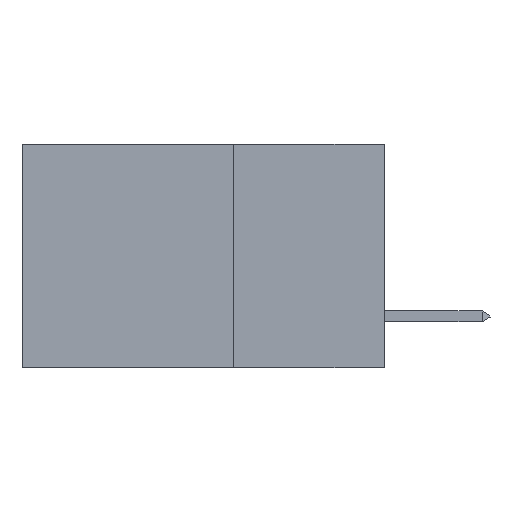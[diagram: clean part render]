
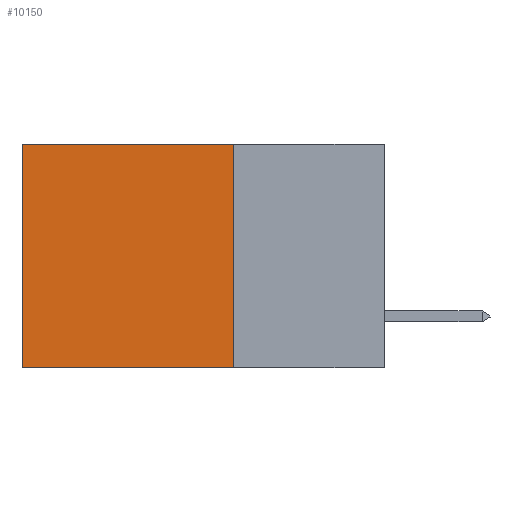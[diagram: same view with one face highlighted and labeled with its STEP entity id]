
A CAD part, left-side view. The second image highlights one B-rep face of the part: STEP entity #10150.
In plain terms, the highlighted planar face has unit normal (-1, 0, 0).
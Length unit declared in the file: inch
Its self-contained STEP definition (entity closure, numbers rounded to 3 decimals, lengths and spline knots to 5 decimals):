
#1330 = CARTESIAN_POINT ( 'NONE',  ( 0.2875, 0.25, 0. ) ) ;
#1349 = VERTEX_POINT ( 'NONE', #18195 ) ;
#1393 = ORIENTED_EDGE ( 'NONE', *, *, #1537, .T. ) ;
#1537 = EDGE_CURVE ( 'NONE', #9768, #7274, #18006, .T. ) ;
#1590 = DIRECTION ( 'NONE',  ( 0., 1., 0. ) ) ;
#2184 = AXIS2_PLACEMENT_3D ( 'NONE', #16130, #9643, #20059 ) ;
#3835 = CARTESIAN_POINT ( 'NONE',  ( 0.2875, 0.25, 0. ) ) ;
#4248 = LINE ( 'NONE', #23626, #9176 ) ;
#4972 = VECTOR ( 'NONE', #26073, 39.37008 ) ;
#5607 = LINE ( 'NONE', #13939, #13127 ) ;
#7274 = VERTEX_POINT ( 'NONE', #18764 ) ;
#8021 = CARTESIAN_POINT ( 'NONE',  ( 0.2875, 0.6, -0.37 ) ) ;
#8277 = EDGE_CURVE ( 'NONE', #7274, #23681, #22443, .T. ) ;
#9176 = VECTOR ( 'NONE', #21908, 39.37008 ) ;
#9643 = DIRECTION ( 'NONE',  ( 1., 0., 0. ) ) ;
#9768 = VERTEX_POINT ( 'NONE', #1330 ) ;
#10150 = ADVANCED_FACE ( 'NONE', ( #24324 ), #26459, .F. ) ;
#10939 = EDGE_LOOP ( 'NONE', ( #15157, #27144, #17195, #1393 ) ) ;
#11761 = DIRECTION ( 'NONE',  ( 0., 0., -1. ) ) ;
#13127 = VECTOR ( 'NONE', #11761, 39.37008 ) ;
#13939 = CARTESIAN_POINT ( 'NONE',  ( 0.2875, 0.25, 0. ) ) ;
#15157 = ORIENTED_EDGE ( 'NONE', *, *, #8277, .T. ) ;
#15782 = EDGE_CURVE ( 'NONE', #9768, #1349, #5607, .T. ) ;
#16130 = CARTESIAN_POINT ( 'NONE',  ( 0.2875, 0.25, 0. ) ) ;
#16409 = EDGE_CURVE ( 'NONE', #1349, #23681, #4248, .T. ) ;
#17195 = ORIENTED_EDGE ( 'NONE', *, *, #15782, .F. ) ;
#17652 = VECTOR ( 'NONE', #1590, 39.37008 ) ;
#18006 = LINE ( 'NONE', #3835, #17652 ) ;
#18195 = CARTESIAN_POINT ( 'NONE',  ( 0.2875, 0.25, -0.37 ) ) ;
#18764 = CARTESIAN_POINT ( 'NONE',  ( 0.2875, 0.6, 0. ) ) ;
#19385 = CARTESIAN_POINT ( 'NONE',  ( 0.2875, 0.6, 0. ) ) ;
#20059 = DIRECTION ( 'NONE',  ( 0., 0., -1. ) ) ;
#21908 = DIRECTION ( 'NONE',  ( 0., 1., 0. ) ) ;
#22443 = LINE ( 'NONE', #19385, #4972 ) ;
#23626 = CARTESIAN_POINT ( 'NONE',  ( 0.2875, 0.25, -0.37 ) ) ;
#23681 = VERTEX_POINT ( 'NONE', #8021 ) ;
#24324 = FACE_OUTER_BOUND ( 'NONE', #10939, .T. ) ;
#26073 = DIRECTION ( 'NONE',  ( 0., 0., -1. ) ) ;
#26459 = PLANE ( 'NONE',  #2184 ) ;
#27144 = ORIENTED_EDGE ( 'NONE', *, *, #16409, .F. ) ;
